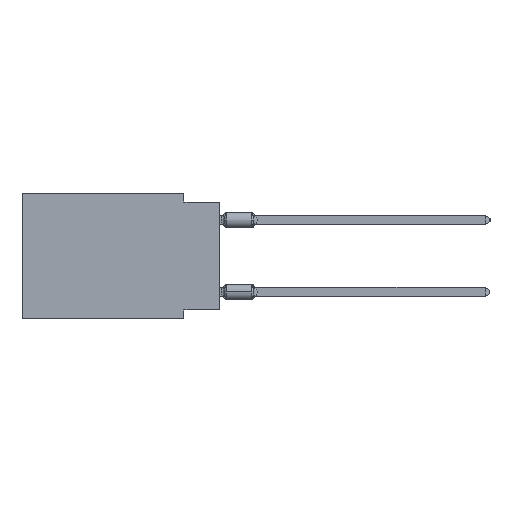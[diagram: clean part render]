
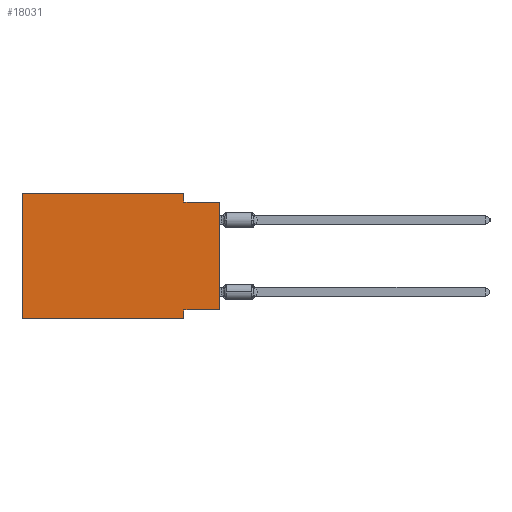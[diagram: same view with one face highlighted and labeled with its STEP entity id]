
A CAD part, left-side view. The second image highlights one B-rep face of the part: STEP entity #18031.
In plain terms, the highlighted planar face has unit normal (-1, 0, 0).
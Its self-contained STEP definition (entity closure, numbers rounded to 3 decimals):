
#484 = VECTOR ( 'NONE', #1101, 1000. ) ;
#673 = CARTESIAN_POINT ( 'NONE',  ( 0., 0., 0. ) ) ;
#1101 = DIRECTION ( 'NONE',  ( 0., 0., -1. ) ) ;
#1130 = CARTESIAN_POINT ( 'NONE',  ( 0., 0., -0.635 ) ) ;
#1568 = LINE ( 'NONE', #28590, #18602 ) ;
#1634 = EDGE_CURVE ( 'NONE', #4571, #5264, #30436, .T. ) ;
#1796 = CARTESIAN_POINT ( 'NONE',  ( 0., 13.97, 0. ) ) ;
#2910 = VERTEX_POINT ( 'NONE', #15190 ) ;
#3679 = DIRECTION ( 'NONE',  ( 0., -1., 0. ) ) ;
#4200 = VECTOR ( 'NONE', #11020, 1000. ) ;
#4348 = VERTEX_POINT ( 'NONE', #13092 ) ;
#4571 = VERTEX_POINT ( 'NONE', #29557 ) ;
#4588 = DIRECTION ( 'NONE',  ( 0., 1., 0. ) ) ;
#4720 = DIRECTION ( 'NONE',  ( 0., 0., -1. ) ) ;
#5264 = VERTEX_POINT ( 'NONE', #28197 ) ;
#5357 = ORIENTED_EDGE ( 'NONE', *, *, #6841, .F. ) ;
#5697 = ORIENTED_EDGE ( 'NONE', *, *, #1634, .F. ) ;
#6564 = ORIENTED_EDGE ( 'NONE', *, *, #18939, .F. ) ;
#6841 = EDGE_CURVE ( 'NONE', #4348, #12712, #19813, .T. ) ;
#8135 = LINE ( 'NONE', #673, #13972 ) ;
#8565 = CARTESIAN_POINT ( 'NONE',  ( 0., 2.54, 0. ) ) ;
#8694 = CARTESIAN_POINT ( 'NONE',  ( 0., 0., -8.255 ) ) ;
#9069 = VERTEX_POINT ( 'NONE', #8694 ) ;
#9256 = AXIS2_PLACEMENT_3D ( 'NONE', #29788, #27041, #4720 ) ;
#10100 = CARTESIAN_POINT ( 'NONE',  ( 0., 13.97, 0. ) ) ;
#11020 = DIRECTION ( 'NONE',  ( 0., -1., 0. ) ) ;
#12712 = VERTEX_POINT ( 'NONE', #18194 ) ;
#12854 = ORIENTED_EDGE ( 'NONE', *, *, #14056, .T. ) ;
#13092 = CARTESIAN_POINT ( 'NONE',  ( 0., 13.97, 0. ) ) ;
#13480 = CARTESIAN_POINT ( 'NONE',  ( 0., 2.54, -8.89 ) ) ;
#13692 = VERTEX_POINT ( 'NONE', #14866 ) ;
#13972 = VECTOR ( 'NONE', #15717, 1000. ) ;
#14056 = EDGE_CURVE ( 'NONE', #2910, #14300, #1568, .T. ) ;
#14300 = VERTEX_POINT ( 'NONE', #13480 ) ;
#14866 = CARTESIAN_POINT ( 'NONE',  ( 0., 2.54, -8.255 ) ) ;
#15190 = CARTESIAN_POINT ( 'NONE',  ( 0., 13.97, -8.89 ) ) ;
#15711 = EDGE_LOOP ( 'NONE', ( #21447, #5697, #6564, #5357, #19080, #12854, #17645, #30972 ) ) ;
#15717 = DIRECTION ( 'NONE',  ( 0., 0., 1. ) ) ;
#16895 = CARTESIAN_POINT ( 'NONE',  ( 0., 0., -8.255 ) ) ;
#17645 = ORIENTED_EDGE ( 'NONE', *, *, #24776, .F. ) ;
#18031 = ADVANCED_FACE ( 'NONE', ( #26887 ), #29480, .F. ) ;
#18194 = CARTESIAN_POINT ( 'NONE',  ( 0., 2.54, 0. ) ) ;
#18602 = VECTOR ( 'NONE', #3679, 1000. ) ;
#18939 = EDGE_CURVE ( 'NONE', #12712, #4571, #30725, .T. ) ;
#19080 = ORIENTED_EDGE ( 'NONE', *, *, #21576, .F. ) ;
#19408 = VECTOR ( 'NONE', #20136, 1000. ) ;
#19413 = VECTOR ( 'NONE', #4588, 1000. ) ;
#19813 = LINE ( 'NONE', #10100, #19408 ) ;
#20136 = DIRECTION ( 'NONE',  ( 0., -1., 0. ) ) ;
#21397 = EDGE_CURVE ( 'NONE', #9069, #5264, #8135, .T. ) ;
#21447 = ORIENTED_EDGE ( 'NONE', *, *, #21397, .T. ) ;
#21576 = EDGE_CURVE ( 'NONE', #2910, #4348, #26389, .T. ) ;
#23818 = DIRECTION ( 'NONE',  ( 0., 0., 1. ) ) ;
#24776 = EDGE_CURVE ( 'NONE', #13692, #14300, #26643, .T. ) ;
#26333 = DIRECTION ( 'NONE',  ( 0., 0., -1. ) ) ;
#26352 = VECTOR ( 'NONE', #23818, 1000. ) ;
#26389 = LINE ( 'NONE', #1796, #26352 ) ;
#26643 = LINE ( 'NONE', #29081, #31697 ) ;
#26887 = FACE_OUTER_BOUND ( 'NONE', #15711, .T. ) ;
#27041 = DIRECTION ( 'NONE',  ( 1., 0., 0. ) ) ;
#27218 = LINE ( 'NONE', #16895, #19413 ) ;
#27962 = EDGE_CURVE ( 'NONE', #9069, #13692, #27218, .T. ) ;
#28197 = CARTESIAN_POINT ( 'NONE',  ( 0., 0., -0.635 ) ) ;
#28590 = CARTESIAN_POINT ( 'NONE',  ( 0., 13.97, -8.89 ) ) ;
#29081 = CARTESIAN_POINT ( 'NONE',  ( 0., 2.54, -8.89 ) ) ;
#29480 = PLANE ( 'NONE',  #9256 ) ;
#29557 = CARTESIAN_POINT ( 'NONE',  ( 0., 2.54, -0.635 ) ) ;
#29788 = CARTESIAN_POINT ( 'NONE',  ( 0., 13.97, 0. ) ) ;
#30436 = LINE ( 'NONE', #1130, #4200 ) ;
#30725 = LINE ( 'NONE', #8565, #484 ) ;
#30972 = ORIENTED_EDGE ( 'NONE', *, *, #27962, .F. ) ;
#31697 = VECTOR ( 'NONE', #26333, 1000. ) ;
